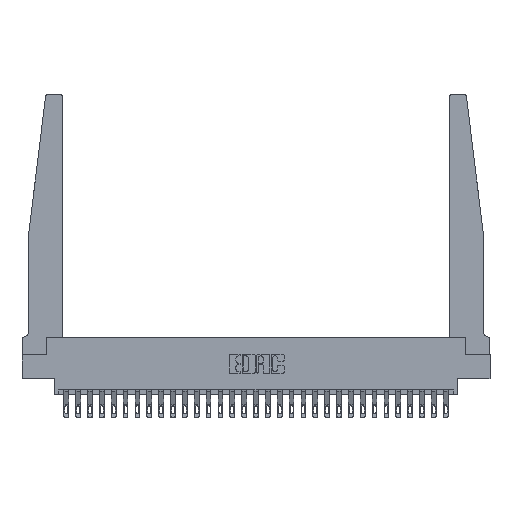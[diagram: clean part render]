
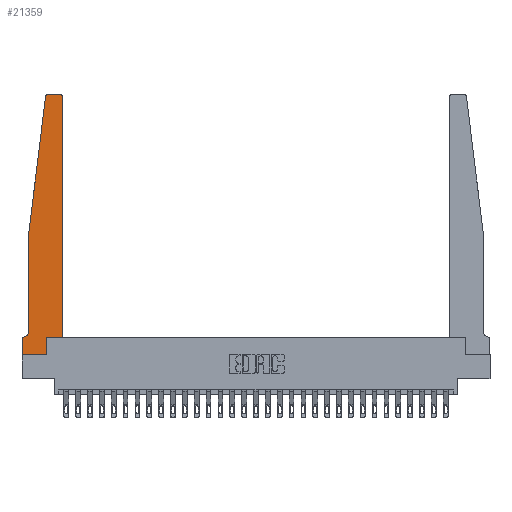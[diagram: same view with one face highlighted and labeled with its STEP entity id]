
A CAD part, top view. The second image highlights one B-rep face of the part: STEP entity #21359.
In plain terms, the highlighted planar face has unit normal (0, 0, 1).
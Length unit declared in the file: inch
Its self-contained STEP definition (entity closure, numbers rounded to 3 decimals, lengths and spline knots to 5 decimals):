
#360 = CARTESIAN_POINT ( 'NONE',  ( 0.24675, 2.72367, 0.37 ) ) ;
#1117 = CARTESIAN_POINT ( 'NONE',  ( 0., 0., 0.37 ) ) ;
#1487 = DIRECTION ( 'NONE',  ( -1., 0., 0. ) ) ;
#1674 = CARTESIAN_POINT ( 'NONE',  ( 0.425, 0.18, 0.37 ) ) ;
#1764 = DIRECTION ( 'NONE',  ( 1., 0., 0. ) ) ;
#1823 = LINE ( 'NONE', #1674, #12166 ) ;
#2023 = DIRECTION ( 'NONE',  ( 0., -1., 0. ) ) ;
#2284 = FACE_OUTER_BOUND ( 'NONE', #26963, .T. ) ;
#2733 = CIRCLE ( 'NONE', #11868, 0.03 ) ;
#3045 = EDGE_CURVE ( 'NONE', #14896, #19949, #11144, .T. ) ;
#3846 = ORIENTED_EDGE ( 'NONE', *, *, #4609, .T. ) ;
#3988 = ORIENTED_EDGE ( 'NONE', *, *, #5290, .T. ) ;
#4461 = ORIENTED_EDGE ( 'NONE', *, *, #21360, .T. ) ;
#4475 = LINE ( 'NONE', #13210, #12286 ) ;
#4609 = EDGE_CURVE ( 'NONE', #26573, #14896, #2733, .T. ) ;
#4702 = ORIENTED_EDGE ( 'NONE', *, *, #12681, .T. ) ;
#4789 = CARTESIAN_POINT ( 'NONE',  ( 0., 0., 0.37 ) ) ;
#5023 = CARTESIAN_POINT ( 'NONE',  ( 0.27653, 2.75, 0.37 ) ) ;
#5290 = EDGE_CURVE ( 'NONE', #7961, #27142, #6896, .T. ) ;
#5416 = VECTOR ( 'NONE', #13865, 39.37008 ) ;
#6102 = CARTESIAN_POINT ( 'NONE',  ( 0.395, 2.75, 0.37 ) ) ;
#6598 = AXIS2_PLACEMENT_3D ( 'NONE', #7393, #16137, #1487 ) ;
#6738 = DIRECTION ( 'NONE',  ( 1., 0., 0. ) ) ;
#6834 = ORIENTED_EDGE ( 'NONE', *, *, #14995, .T. ) ;
#6896 = CIRCLE ( 'NONE', #20596, 0.03 ) ;
#7014 = CARTESIAN_POINT ( 'NONE',  ( 0.015, 0.1875, 0.37 ) ) ;
#7393 = CARTESIAN_POINT ( 'NONE',  ( 0.015, 0.2375, 0.37 ) ) ;
#7588 = ORIENTED_EDGE ( 'NONE', *, *, #20884, .T. ) ;
#7885 = LINE ( 'NONE', #25391, #14924 ) ;
#7931 = ORIENTED_EDGE ( 'NONE', *, *, #24700, .T. ) ;
#7961 = VERTEX_POINT ( 'NONE', #17748 ) ;
#8581 = AXIS2_PLACEMENT_3D ( 'NONE', #11042, #15005, #6738 ) ;
#9009 = VERTEX_POINT ( 'NONE', #1117 ) ;
#9406 = CARTESIAN_POINT ( 'NONE',  ( 0.425, 0.18, 0.37 ) ) ;
#9559 = VECTOR ( 'NONE', #12319, 39.37008 ) ;
#10602 = VERTEX_POINT ( 'NONE', #13306 ) ;
#10603 = LINE ( 'NONE', #19355, #26478 ) ;
#10634 = DIRECTION ( 'NONE',  ( 0., 0., 1. ) ) ;
#11042 = CARTESIAN_POINT ( 'NONE',  ( 0., 0.1875, 0.37 ) ) ;
#11144 = LINE ( 'NONE', #16634, #9559 ) ;
#11313 = CARTESIAN_POINT ( 'NONE',  ( 0.065, 1.25, 0.37 ) ) ;
#11581 = ORIENTED_EDGE ( 'NONE', *, *, #3045, .T. ) ;
#11868 = AXIS2_PLACEMENT_3D ( 'NONE', #27892, #10634, #25996 ) ;
#12166 = VECTOR ( 'NONE', #25370, 39.37008 ) ;
#12286 = VECTOR ( 'NONE', #2023, 39.37008 ) ;
#12319 = DIRECTION ( 'NONE',  ( -0.122, -0.992, 0. ) ) ;
#12681 = EDGE_CURVE ( 'NONE', #10602, #27056, #7885, .T. ) ;
#12807 = CARTESIAN_POINT ( 'NONE',  ( 0.065, 0.1875, 0.37 ) ) ;
#12943 = CARTESIAN_POINT ( 'NONE',  ( 0.395, 2.72, 0.37 ) ) ;
#12954 = LINE ( 'NONE', #12807, #19349 ) ;
#13171 = PLANE ( 'NONE',  #8581 ) ;
#13210 = CARTESIAN_POINT ( 'NONE',  ( 0.065, 1.25, 0.37 ) ) ;
#13306 = CARTESIAN_POINT ( 'NONE',  ( 0.2605, 0.18, 0.37 ) ) ;
#13456 = CARTESIAN_POINT ( 'NONE',  ( 0.25, 2.75, 0.37 ) ) ;
#13511 = DIRECTION ( 'NONE',  ( 0., -1., 0. ) ) ;
#13865 = DIRECTION ( 'NONE',  ( -1., 0., 0. ) ) ;
#14519 = ORIENTED_EDGE ( 'NONE', *, *, #28039, .T. ) ;
#14539 = VERTEX_POINT ( 'NONE', #18630 ) ;
#14553 = DIRECTION ( 'NONE',  ( 1., 0., 0. ) ) ;
#14896 = VERTEX_POINT ( 'NONE', #360 ) ;
#14924 = VECTOR ( 'NONE', #25679, 39.37008 ) ;
#14995 = EDGE_CURVE ( 'NONE', #14539, #25243, #15249, .T. ) ;
#15005 = DIRECTION ( 'NONE',  ( 0., 0., 1. ) ) ;
#15090 = DIRECTION ( 'NONE',  ( -1., 0., 0. ) ) ;
#15249 = CIRCLE ( 'NONE', #6598, 0.05 ) ;
#15444 = LINE ( 'NONE', #13456, #5416 ) ;
#16137 = DIRECTION ( 'NONE',  ( 0., 0., -1. ) ) ;
#16548 = VECTOR ( 'NONE', #13511, 39.37008 ) ;
#16634 = CARTESIAN_POINT ( 'NONE',  ( 0.065, 1.25, 0.37 ) ) ;
#17748 = CARTESIAN_POINT ( 'NONE',  ( 0.425, 2.72, 0.37 ) ) ;
#18332 = CARTESIAN_POINT ( 'NONE',  ( 0., 0.1875, 0.37 ) ) ;
#18630 = CARTESIAN_POINT ( 'NONE',  ( 0.065, 0.2375, 0.37 ) ) ;
#19349 = VECTOR ( 'NONE', #15090, 39.37008 ) ;
#19355 = CARTESIAN_POINT ( 'NONE',  ( 0.2605, 0.18, 0.37 ) ) ;
#19766 = EDGE_CURVE ( 'NONE', #27056, #7961, #1823, .T. ) ;
#19949 = VERTEX_POINT ( 'NONE', #11313 ) ;
#19989 = ORIENTED_EDGE ( 'NONE', *, *, #19766, .T. ) ;
#20596 = AXIS2_PLACEMENT_3D ( 'NONE', #12943, #28214, #1764 ) ;
#20884 = EDGE_CURVE ( 'NONE', #19949, #14539, #4475, .T. ) ;
#21359 = ADVANCED_FACE ( 'NONE', ( #2284 ), #13171, .T. ) ;
#21360 = EDGE_CURVE ( 'NONE', #27142, #26573, #15444, .T. ) ;
#22576 = EDGE_CURVE ( 'NONE', #25627, #10602, #10603, .T. ) ;
#23145 = ORIENTED_EDGE ( 'NONE', *, *, #25431, .T. ) ;
#24039 = CARTESIAN_POINT ( 'NONE',  ( 0.2605, 0., 0.37 ) ) ;
#24086 = DIRECTION ( 'NONE',  ( 0., 1., 0. ) ) ;
#24429 = LINE ( 'NONE', #4789, #16548 ) ;
#24700 = EDGE_CURVE ( 'NONE', #25243, #26685, #12954, .T. ) ;
#25078 = LINE ( 'NONE', #25492, #25595 ) ;
#25243 = VERTEX_POINT ( 'NONE', #7014 ) ;
#25370 = DIRECTION ( 'NONE',  ( 0., 1., 0. ) ) ;
#25391 = CARTESIAN_POINT ( 'NONE',  ( 0.425, 0.18, 0.37 ) ) ;
#25431 = EDGE_CURVE ( 'NONE', #9009, #25627, #25078, .T. ) ;
#25492 = CARTESIAN_POINT ( 'NONE',  ( 0., 0., 0.37 ) ) ;
#25595 = VECTOR ( 'NONE', #14553, 39.37008 ) ;
#25627 = VERTEX_POINT ( 'NONE', #24039 ) ;
#25679 = DIRECTION ( 'NONE',  ( 1., 0., 0. ) ) ;
#25996 = DIRECTION ( 'NONE',  ( 1., 0., 0. ) ) ;
#26478 = VECTOR ( 'NONE', #24086, 39.37008 ) ;
#26573 = VERTEX_POINT ( 'NONE', #5023 ) ;
#26685 = VERTEX_POINT ( 'NONE', #18332 ) ;
#26933 = ORIENTED_EDGE ( 'NONE', *, *, #22576, .T. ) ;
#26963 = EDGE_LOOP ( 'NONE', ( #4461, #3846, #11581, #7588, #6834, #7931, #14519, #23145, #26933, #4702, #19989, #3988 ) ) ;
#27056 = VERTEX_POINT ( 'NONE', #9406 ) ;
#27142 = VERTEX_POINT ( 'NONE', #6102 ) ;
#27892 = CARTESIAN_POINT ( 'NONE',  ( 0.27653, 2.72, 0.37 ) ) ;
#28039 = EDGE_CURVE ( 'NONE', #26685, #9009, #24429, .T. ) ;
#28214 = DIRECTION ( 'NONE',  ( 0., 0., 1. ) ) ;
